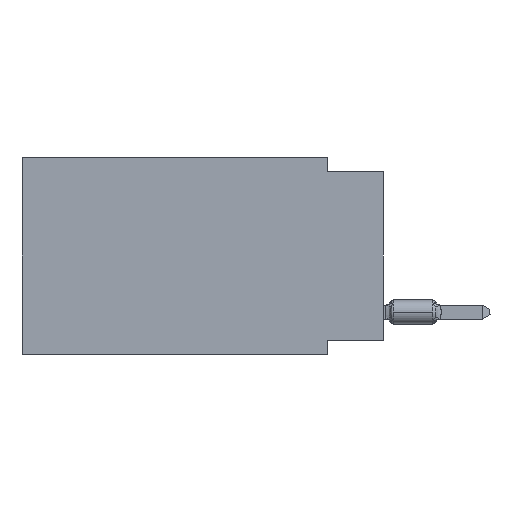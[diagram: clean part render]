
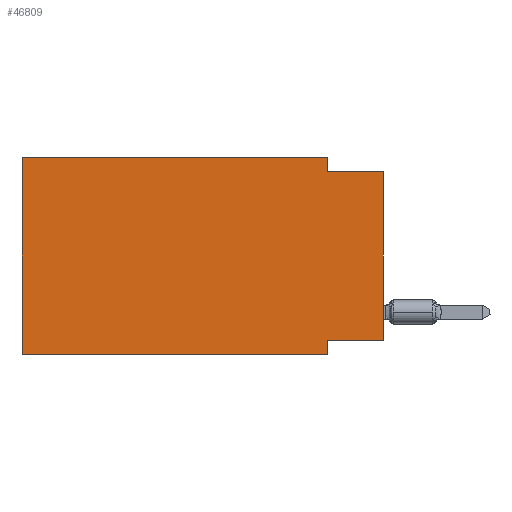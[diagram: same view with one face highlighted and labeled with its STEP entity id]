
A CAD part, left-side view. The second image highlights one B-rep face of the part: STEP entity #46809.
In plain terms, the highlighted planar face has unit normal (-1, 0, 0).
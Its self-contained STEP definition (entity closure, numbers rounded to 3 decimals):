
#1300 = EDGE_LOOP ( 'NONE', ( #79229, #45364, #115764, #70326, #97019, #11857, #33698, #40472 ) ) ;
#3985 = LINE ( 'NONE', #49267, #32085 ) ;
#5615 = VECTOR ( 'NONE', #44838, 1000. ) ;
#5929 = VERTEX_POINT ( 'NONE', #49603 ) ;
#11857 = ORIENTED_EDGE ( 'NONE', *, *, #69975, .T. ) ;
#12961 = EDGE_CURVE ( 'NONE', #97175, #50211, #87889, .T. ) ;
#13308 = VECTOR ( 'NONE', #113518, 1000. ) ;
#14023 = CARTESIAN_POINT ( 'NONE',  ( 0., 0., -0.635 ) ) ;
#14757 = LINE ( 'NONE', #61822, #105573 ) ;
#15811 = CARTESIAN_POINT ( 'NONE',  ( 0., 0., -8.255 ) ) ;
#16957 = DIRECTION ( 'NONE',  ( 0., 1., 0. ) ) ;
#19353 = VERTEX_POINT ( 'NONE', #28879 ) ;
#22064 = VERTEX_POINT ( 'NONE', #106489 ) ;
#23131 = CARTESIAN_POINT ( 'NONE',  ( 0., 2.54, -8.255 ) ) ;
#24293 = DIRECTION ( 'NONE',  ( 0., -1., 0. ) ) ;
#28879 = CARTESIAN_POINT ( 'NONE',  ( 0., 2.54, -0.635 ) ) ;
#29267 = FACE_OUTER_BOUND ( 'NONE', #1300, .T. ) ;
#32085 = VECTOR ( 'NONE', #77840, 1000. ) ;
#32863 = CARTESIAN_POINT ( 'NONE',  ( 0., 2.54, 0. ) ) ;
#33698 = ORIENTED_EDGE ( 'NONE', *, *, #74193, .F. ) ;
#40472 = ORIENTED_EDGE ( 'NONE', *, *, #62271, .F. ) ;
#41422 = CARTESIAN_POINT ( 'NONE',  ( 0., 16.383, 0. ) ) ;
#44353 = LINE ( 'NONE', #53277, #63665 ) ;
#44838 = DIRECTION ( 'NONE',  ( 0., 0., 1. ) ) ;
#45364 = ORIENTED_EDGE ( 'NONE', *, *, #82847, .F. ) ;
#45420 = DIRECTION ( 'NONE',  ( 0., 0., -1. ) ) ;
#46809 = ADVANCED_FACE ( 'NONE', ( #29267 ), #93012, .F. ) ;
#48643 = EDGE_CURVE ( 'NONE', #92337, #5929, #53176, .T. ) ;
#49267 = CARTESIAN_POINT ( 'NONE',  ( 0., 2.54, 0. ) ) ;
#49603 = CARTESIAN_POINT ( 'NONE',  ( 0., 0., -0.635 ) ) ;
#50211 = VERTEX_POINT ( 'NONE', #114612 ) ;
#51493 = AXIS2_PLACEMENT_3D ( 'NONE', #65617, #57242, #56666 ) ;
#53176 = LINE ( 'NONE', #98475, #5615 ) ;
#53277 = CARTESIAN_POINT ( 'NONE',  ( 0., 16.383, -8.89 ) ) ;
#56666 = DIRECTION ( 'NONE',  ( 0., 0., -1. ) ) ;
#57242 = DIRECTION ( 'NONE',  ( 1., 0., 0. ) ) ;
#58650 = EDGE_CURVE ( 'NONE', #50211, #87865, #14757, .T. ) ;
#58715 = DIRECTION ( 'NONE',  ( 0., -1., 0. ) ) ;
#61822 = CARTESIAN_POINT ( 'NONE',  ( 0., 16.383, 0. ) ) ;
#62271 = EDGE_CURVE ( 'NONE', #92337, #74936, #81309, .T. ) ;
#63665 = VECTOR ( 'NONE', #109263, 1000. ) ;
#65617 = CARTESIAN_POINT ( 'NONE',  ( 0., 16.383, 0. ) ) ;
#69975 = EDGE_CURVE ( 'NONE', #97175, #22064, #44353, .T. ) ;
#70326 = ORIENTED_EDGE ( 'NONE', *, *, #58650, .F. ) ;
#72236 = CARTESIAN_POINT ( 'NONE',  ( 0., 2.54, -8.89 ) ) ;
#74193 = EDGE_CURVE ( 'NONE', #74936, #22064, #109175, .T. ) ;
#74936 = VERTEX_POINT ( 'NONE', #23131 ) ;
#76048 = VECTOR ( 'NONE', #58715, 1000. ) ;
#77840 = DIRECTION ( 'NONE',  ( 0., 0., -1. ) ) ;
#79229 = ORIENTED_EDGE ( 'NONE', *, *, #48643, .T. ) ;
#81309 = LINE ( 'NONE', #15811, #89294 ) ;
#82847 = EDGE_CURVE ( 'NONE', #19353, #5929, #104013, .T. ) ;
#86848 = VECTOR ( 'NONE', #45420, 1000. ) ;
#87865 = VERTEX_POINT ( 'NONE', #32863 ) ;
#87889 = LINE ( 'NONE', #41422, #13308 ) ;
#88724 = EDGE_CURVE ( 'NONE', #87865, #19353, #3985, .T. ) ;
#89294 = VECTOR ( 'NONE', #16957, 1000. ) ;
#92337 = VERTEX_POINT ( 'NONE', #100417 ) ;
#93012 = PLANE ( 'NONE',  #51493 ) ;
#97019 = ORIENTED_EDGE ( 'NONE', *, *, #12961, .F. ) ;
#97175 = VERTEX_POINT ( 'NONE', #102019 ) ;
#98475 = CARTESIAN_POINT ( 'NONE',  ( 0., 0., 0. ) ) ;
#100417 = CARTESIAN_POINT ( 'NONE',  ( 0., 0., -8.255 ) ) ;
#102019 = CARTESIAN_POINT ( 'NONE',  ( 0., 16.383, -8.89 ) ) ;
#104013 = LINE ( 'NONE', #14023, #76048 ) ;
#105573 = VECTOR ( 'NONE', #24293, 1000. ) ;
#106489 = CARTESIAN_POINT ( 'NONE',  ( 0., 2.54, -8.89 ) ) ;
#109175 = LINE ( 'NONE', #72236, #86848 ) ;
#109263 = DIRECTION ( 'NONE',  ( 0., -1., 0. ) ) ;
#113518 = DIRECTION ( 'NONE',  ( 0., 0., 1. ) ) ;
#114612 = CARTESIAN_POINT ( 'NONE',  ( 0., 16.383, 0. ) ) ;
#115764 = ORIENTED_EDGE ( 'NONE', *, *, #88724, .F. ) ;
